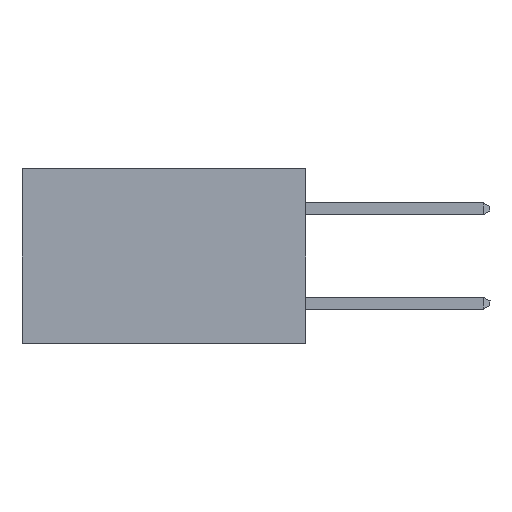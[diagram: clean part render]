
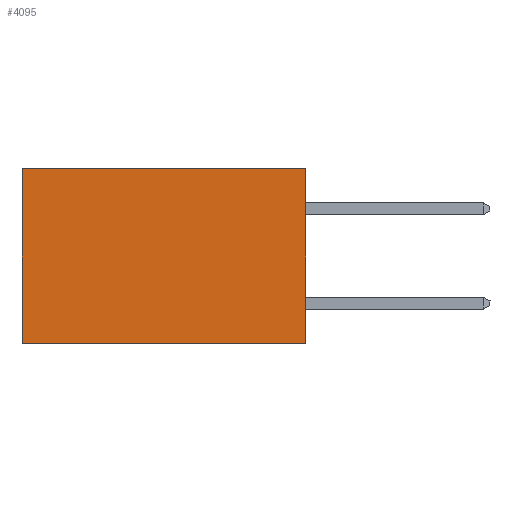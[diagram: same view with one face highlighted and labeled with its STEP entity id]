
A CAD part, left-side view. The second image highlights one B-rep face of the part: STEP entity #4095.
In plain terms, the highlighted planar face has unit normal (-1, 0, 0).
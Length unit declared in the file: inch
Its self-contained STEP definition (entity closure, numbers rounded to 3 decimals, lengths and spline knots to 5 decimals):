
#2 = EDGE_CURVE ( 'NONE', #2143, #7124, #6352, .T. ) ;
#712 = DIRECTION ( 'NONE',  ( 0., 0., -1. ) ) ;
#1349 = AXIS2_PLACEMENT_3D ( 'NONE', #14786, #14270, #14242 ) ;
#1391 = CARTESIAN_POINT ( 'NONE',  ( 0.2615, 0., -0.37 ) ) ;
#1439 = VERTEX_POINT ( 'NONE', #14505 ) ;
#1643 = LINE ( 'NONE', #1391, #13340 ) ;
#1681 = EDGE_CURVE ( 'NONE', #7124, #10431, #5327, .T. ) ;
#2143 = VERTEX_POINT ( 'NONE', #7161 ) ;
#3035 = VECTOR ( 'NONE', #6652, 39.37008 ) ;
#3438 = VECTOR ( 'NONE', #9324, 39.37008 ) ;
#4095 = ADVANCED_FACE ( 'NONE', ( #9792 ), #14303, .F. ) ;
#4562 = EDGE_CURVE ( 'NONE', #2143, #1439, #1643, .T. ) ;
#4760 = ORIENTED_EDGE ( 'NONE', *, *, #4562, .F. ) ;
#5042 = CARTESIAN_POINT ( 'NONE',  ( 0.2615, 0.6, -0.37 ) ) ;
#5327 = LINE ( 'NONE', #8553, #8018 ) ;
#5383 = EDGE_LOOP ( 'NONE', ( #14454, #9049, #4760, #9410 ) ) ;
#6352 = LINE ( 'NONE', #6763, #3035 ) ;
#6652 = DIRECTION ( 'NONE',  ( 0., 1., 0. ) ) ;
#6763 = CARTESIAN_POINT ( 'NONE',  ( 0.2615, 0., 0. ) ) ;
#7124 = VERTEX_POINT ( 'NONE', #11396 ) ;
#7161 = CARTESIAN_POINT ( 'NONE',  ( 0.2615, 0., 0. ) ) ;
#8018 = VECTOR ( 'NONE', #8590, 39.37008 ) ;
#8553 = CARTESIAN_POINT ( 'NONE',  ( 0.2615, 0.6, -0.37 ) ) ;
#8590 = DIRECTION ( 'NONE',  ( 0., 0., -1. ) ) ;
#9049 = ORIENTED_EDGE ( 'NONE', *, *, #9234, .F. ) ;
#9234 = EDGE_CURVE ( 'NONE', #1439, #10431, #9358, .T. ) ;
#9245 = CARTESIAN_POINT ( 'NONE',  ( 0.2615, 0., -0.37 ) ) ;
#9324 = DIRECTION ( 'NONE',  ( 0., 1., 0. ) ) ;
#9358 = LINE ( 'NONE', #9245, #3438 ) ;
#9410 = ORIENTED_EDGE ( 'NONE', *, *, #2, .T. ) ;
#9792 = FACE_OUTER_BOUND ( 'NONE', #5383, .T. ) ;
#10431 = VERTEX_POINT ( 'NONE', #5042 ) ;
#11396 = CARTESIAN_POINT ( 'NONE',  ( 0.2615, 0.6, 0. ) ) ;
#13340 = VECTOR ( 'NONE', #712, 39.37008 ) ;
#14242 = DIRECTION ( 'NONE',  ( 0., 0., -1. ) ) ;
#14270 = DIRECTION ( 'NONE',  ( 1., 0., 0. ) ) ;
#14303 = PLANE ( 'NONE',  #1349 ) ;
#14454 = ORIENTED_EDGE ( 'NONE', *, *, #1681, .T. ) ;
#14505 = CARTESIAN_POINT ( 'NONE',  ( 0.2615, 0., -0.37 ) ) ;
#14786 = CARTESIAN_POINT ( 'NONE',  ( 0.2615, 0., -0.37 ) ) ;
